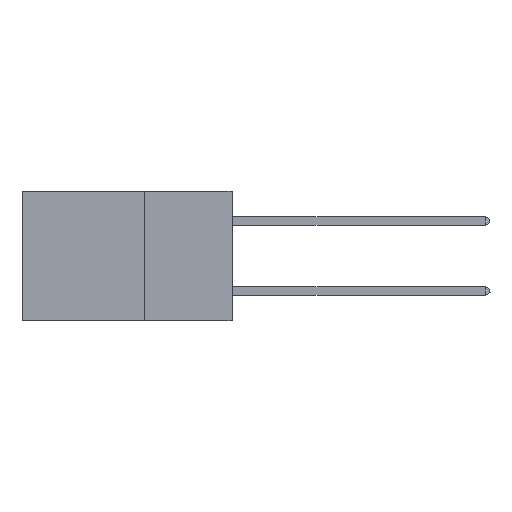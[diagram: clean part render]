
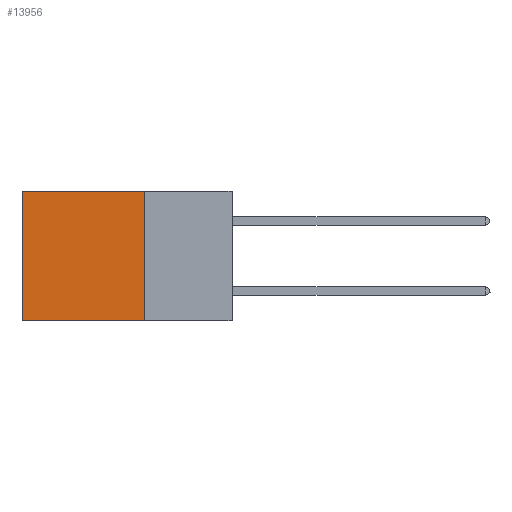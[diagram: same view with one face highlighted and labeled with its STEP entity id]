
A CAD part, left-side view. The second image highlights one B-rep face of the part: STEP entity #13956.
In plain terms, the highlighted planar face has unit normal (-1, 0, 0).
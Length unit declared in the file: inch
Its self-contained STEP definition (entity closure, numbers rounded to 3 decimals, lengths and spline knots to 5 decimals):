
#1157 = VERTEX_POINT ( 'NONE', #4377 ) ;
#1649 = DIRECTION ( 'NONE',  ( 0., 1., 0. ) ) ;
#1826 = CARTESIAN_POINT ( 'NONE',  ( 0.2875, 0.25, -0.37 ) ) ;
#1898 = DIRECTION ( 'NONE',  ( 0., 0., -1. ) ) ;
#2019 = LINE ( 'NONE', #1826, #15370 ) ;
#2211 = CARTESIAN_POINT ( 'NONE',  ( 0.2875, 0.25, 0. ) ) ;
#2318 = DIRECTION ( 'NONE',  ( 0., 0., -1. ) ) ;
#2897 = DIRECTION ( 'NONE',  ( 0., 0., -1. ) ) ;
#3751 = FACE_OUTER_BOUND ( 'NONE', #15506, .T. ) ;
#4377 = CARTESIAN_POINT ( 'NONE',  ( 0.2875, 0.6, 0. ) ) ;
#4720 = DIRECTION ( 'NONE',  ( 0., 1., 0. ) ) ;
#7611 = ORIENTED_EDGE ( 'NONE', *, *, #16258, .F. ) ;
#8131 = ORIENTED_EDGE ( 'NONE', *, *, #12083, .T. ) ;
#8568 = PLANE ( 'NONE',  #18150 ) ;
#9075 = VERTEX_POINT ( 'NONE', #2211 ) ;
#9159 = CARTESIAN_POINT ( 'NONE',  ( 0.2875, 0.25, 0. ) ) ;
#9648 = VECTOR ( 'NONE', #1649, 39.37008 ) ;
#9782 = VERTEX_POINT ( 'NONE', #13480 ) ;
#10846 = LINE ( 'NONE', #13308, #11302 ) ;
#11302 = VECTOR ( 'NONE', #2897, 39.37008 ) ;
#11404 = CARTESIAN_POINT ( 'NONE',  ( 0.2875, 0.25, 0. ) ) ;
#12083 = EDGE_CURVE ( 'NONE', #1157, #14943, #10846, .T. ) ;
#12179 = LINE ( 'NONE', #15191, #17979 ) ;
#12660 = LINE ( 'NONE', #9159, #9648 ) ;
#13262 = EDGE_CURVE ( 'NONE', #9075, #1157, #12660, .T. ) ;
#13308 = CARTESIAN_POINT ( 'NONE',  ( 0.2875, 0.6, 0. ) ) ;
#13480 = CARTESIAN_POINT ( 'NONE',  ( 0.2875, 0.25, -0.37 ) ) ;
#13956 = ADVANCED_FACE ( 'NONE', ( #3751 ), #8568, .F. ) ;
#14393 = EDGE_CURVE ( 'NONE', #9075, #9782, #12179, .T. ) ;
#14558 = ORIENTED_EDGE ( 'NONE', *, *, #13262, .T. ) ;
#14943 = VERTEX_POINT ( 'NONE', #16636 ) ;
#15191 = CARTESIAN_POINT ( 'NONE',  ( 0.2875, 0.25, 0. ) ) ;
#15370 = VECTOR ( 'NONE', #4720, 39.37008 ) ;
#15506 = EDGE_LOOP ( 'NONE', ( #8131, #7611, #18147, #14558 ) ) ;
#16258 = EDGE_CURVE ( 'NONE', #9782, #14943, #2019, .T. ) ;
#16636 = CARTESIAN_POINT ( 'NONE',  ( 0.2875, 0.6, -0.37 ) ) ;
#17387 = DIRECTION ( 'NONE',  ( 1., 0., 0. ) ) ;
#17979 = VECTOR ( 'NONE', #1898, 39.37008 ) ;
#18147 = ORIENTED_EDGE ( 'NONE', *, *, #14393, .F. ) ;
#18150 = AXIS2_PLACEMENT_3D ( 'NONE', #11404, #17387, #2318 ) ;
